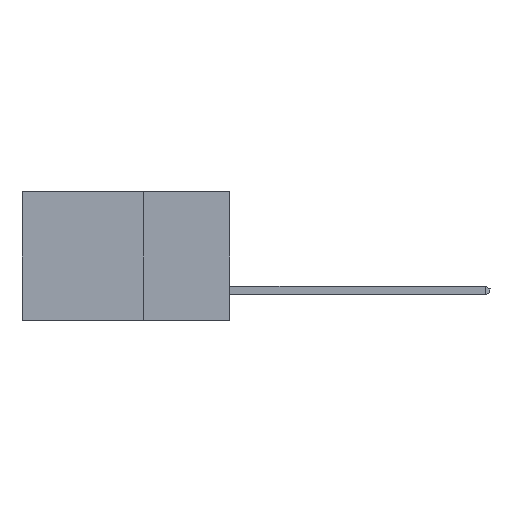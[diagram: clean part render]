
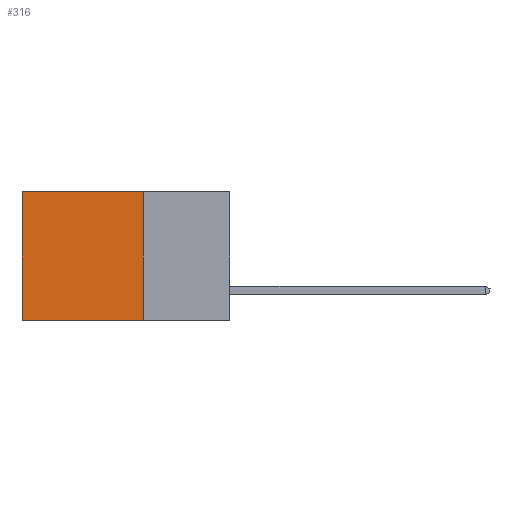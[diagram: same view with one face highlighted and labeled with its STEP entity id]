
A CAD part, left-side view. The second image highlights one B-rep face of the part: STEP entity #316.
In plain terms, the highlighted planar face has unit normal (-1, 0, 0).
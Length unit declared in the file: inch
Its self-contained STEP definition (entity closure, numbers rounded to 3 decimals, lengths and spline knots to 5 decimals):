
#219 = CARTESIAN_POINT ( 'NONE',  ( 0.2615, 0.25, -0.37 ) ) ;
#316 = ADVANCED_FACE ( 'NONE', ( #8544 ), #3019, .F. ) ;
#1018 = ORIENTED_EDGE ( 'NONE', *, *, #8369, .T. ) ;
#1132 = VERTEX_POINT ( 'NONE', #219 ) ;
#1323 = EDGE_LOOP ( 'NONE', ( #7358, #8631, #3568, #1018 ) ) ;
#1418 = CARTESIAN_POINT ( 'NONE',  ( 0.2615, 0.6, -0.37 ) ) ;
#2815 = CARTESIAN_POINT ( 'NONE',  ( 0.2615, 0.6, 0. ) ) ;
#2846 = EDGE_CURVE ( 'NONE', #1132, #9404, #11457, .T. ) ;
#3019 = PLANE ( 'NONE',  #8244 ) ;
#3372 = DIRECTION ( 'NONE',  ( 1., 0., 0. ) ) ;
#3568 = ORIENTED_EDGE ( 'NONE', *, *, #9172, .F. ) ;
#3786 = VECTOR ( 'NONE', #5727, 39.37008 ) ;
#4936 = VERTEX_POINT ( 'NONE', #2815 ) ;
#5451 = CARTESIAN_POINT ( 'NONE',  ( 0.2615, 0.25, -0.37 ) ) ;
#5639 = CARTESIAN_POINT ( 'NONE',  ( 0.2615, 0.6, -0.37 ) ) ;
#5727 = DIRECTION ( 'NONE',  ( 0., 1., 0. ) ) ;
#5941 = LINE ( 'NONE', #1418, #9179 ) ;
#6208 = VERTEX_POINT ( 'NONE', #11094 ) ;
#6334 = VECTOR ( 'NONE', #7924, 39.37008 ) ;
#6463 = VECTOR ( 'NONE', #7889, 39.37008 ) ;
#6490 = EDGE_CURVE ( 'NONE', #4936, #9404, #5941, .T. ) ;
#6912 = DIRECTION ( 'NONE',  ( 0., 0., -1. ) ) ;
#6976 = DIRECTION ( 'NONE',  ( 0., 0., -1. ) ) ;
#7358 = ORIENTED_EDGE ( 'NONE', *, *, #6490, .T. ) ;
#7889 = DIRECTION ( 'NONE',  ( 0., 1., 0. ) ) ;
#7924 = DIRECTION ( 'NONE',  ( 0., 0., -1. ) ) ;
#8197 = LINE ( 'NONE', #5451, #6334 ) ;
#8244 = AXIS2_PLACEMENT_3D ( 'NONE', #8966, #3372, #6976 ) ;
#8369 = EDGE_CURVE ( 'NONE', #6208, #4936, #11130, .T. ) ;
#8544 = FACE_OUTER_BOUND ( 'NONE', #1323, .T. ) ;
#8631 = ORIENTED_EDGE ( 'NONE', *, *, #2846, .F. ) ;
#8966 = CARTESIAN_POINT ( 'NONE',  ( 0.2615, 0.25, -0.37 ) ) ;
#9172 = EDGE_CURVE ( 'NONE', #6208, #1132, #8197, .T. ) ;
#9179 = VECTOR ( 'NONE', #6912, 39.37008 ) ;
#9307 = CARTESIAN_POINT ( 'NONE',  ( 0.2615, 0.25, 0. ) ) ;
#9404 = VERTEX_POINT ( 'NONE', #5639 ) ;
#10622 = CARTESIAN_POINT ( 'NONE',  ( 0.2615, 0.25, -0.37 ) ) ;
#11094 = CARTESIAN_POINT ( 'NONE',  ( 0.2615, 0.25, 0. ) ) ;
#11130 = LINE ( 'NONE', #9307, #3786 ) ;
#11457 = LINE ( 'NONE', #10622, #6463 ) ;
